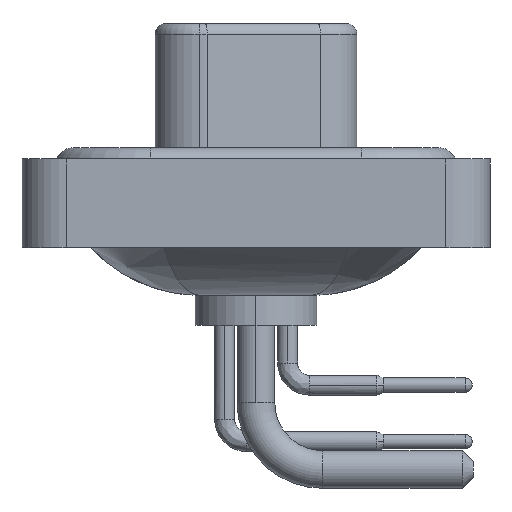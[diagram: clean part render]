
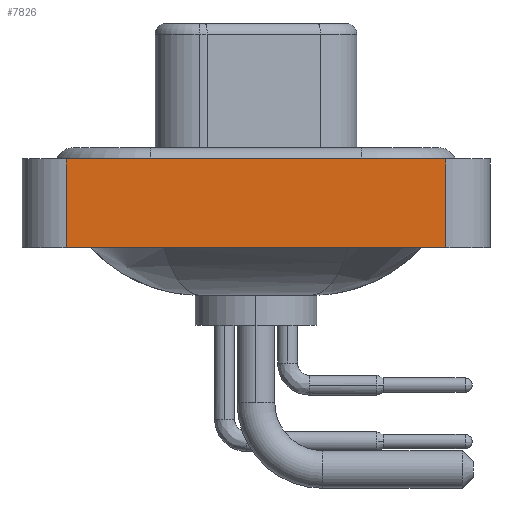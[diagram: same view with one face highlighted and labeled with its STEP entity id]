
A CAD part, left-side view. The second image highlights one B-rep face of the part: STEP entity #7826.
In plain terms, the highlighted planar face has unit normal (-1, 0, 0).
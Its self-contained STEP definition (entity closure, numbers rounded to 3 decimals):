
#916 = DIRECTION ( 'NONE',  ( 0., -1., 0. ) ) ;
#1099 = VERTEX_POINT ( 'NONE', #13042 ) ;
#1100 = EDGE_CURVE ( 'NONE', #1099, #21286, #3601, .T. ) ;
#2170 = FACE_OUTER_BOUND ( 'NONE', #3930, .T. ) ;
#2278 = DIRECTION ( 'NONE',  ( 0., 0., 1. ) ) ;
#3601 = LINE ( 'NONE', #20598, #17471 ) ;
#3930 = EDGE_LOOP ( 'NONE', ( #15878, #4094, #22505, #18860 ) ) ;
#4094 = ORIENTED_EDGE ( 'NONE', *, *, #1100, .F. ) ;
#5117 = CARTESIAN_POINT ( 'NONE',  ( -7.3, -8.55, -3.6 ) ) ;
#5926 = VECTOR ( 'NONE', #19302, 1000. ) ;
#7695 = DIRECTION ( 'NONE',  ( 0., -1., 0. ) ) ;
#7826 = ADVANCED_FACE ( 'NONE', ( #2170 ), #11615, .T. ) ;
#8077 = CARTESIAN_POINT ( 'NONE',  ( -7.3, -8.55, 0.4 ) ) ;
#8120 = LINE ( 'NONE', #9865, #5926 ) ;
#8411 = VECTOR ( 'NONE', #916, 1000. ) ;
#9865 = CARTESIAN_POINT ( 'NONE',  ( -7.3, -8.55, -3.6 ) ) ;
#10079 = DIRECTION ( 'NONE',  ( 0., 0., 1. ) ) ;
#10595 = CARTESIAN_POINT ( 'NONE',  ( -7.3, -8.55, -3.6 ) ) ;
#11615 = PLANE ( 'NONE',  #22421 ) ;
#12175 = VERTEX_POINT ( 'NONE', #13568 ) ;
#12464 = LINE ( 'NONE', #5117, #8411 ) ;
#13042 = CARTESIAN_POINT ( 'NONE',  ( -7.3, 8.55, 0.4 ) ) ;
#13568 = CARTESIAN_POINT ( 'NONE',  ( -7.3, 8.55, -3.6 ) ) ;
#14048 = LINE ( 'NONE', #19271, #19035 ) ;
#15878 = ORIENTED_EDGE ( 'NONE', *, *, #19817, .T. ) ;
#16806 = EDGE_CURVE ( 'NONE', #12175, #16876, #12464, .T. ) ;
#16876 = VERTEX_POINT ( 'NONE', #10595 ) ;
#17471 = VECTOR ( 'NONE', #7695, 1000. ) ;
#18491 = EDGE_CURVE ( 'NONE', #12175, #1099, #14048, .T. ) ;
#18860 = ORIENTED_EDGE ( 'NONE', *, *, #16806, .T. ) ;
#19035 = VECTOR ( 'NONE', #10079, 1000. ) ;
#19271 = CARTESIAN_POINT ( 'NONE',  ( -7.3, 8.55, -3.6 ) ) ;
#19302 = DIRECTION ( 'NONE',  ( 0., 0., 1. ) ) ;
#19638 = DIRECTION ( 'NONE',  ( -1., 0., 0. ) ) ;
#19817 = EDGE_CURVE ( 'NONE', #16876, #21286, #8120, .T. ) ;
#20598 = CARTESIAN_POINT ( 'NONE',  ( -7.3, -8.55, 0.4 ) ) ;
#21286 = VERTEX_POINT ( 'NONE', #8077 ) ;
#22421 = AXIS2_PLACEMENT_3D ( 'NONE', #23482, #19638, #2278 ) ;
#22505 = ORIENTED_EDGE ( 'NONE', *, *, #18491, .F. ) ;
#23482 = CARTESIAN_POINT ( 'NONE',  ( -7.3, -8.55, -3.6 ) ) ;
